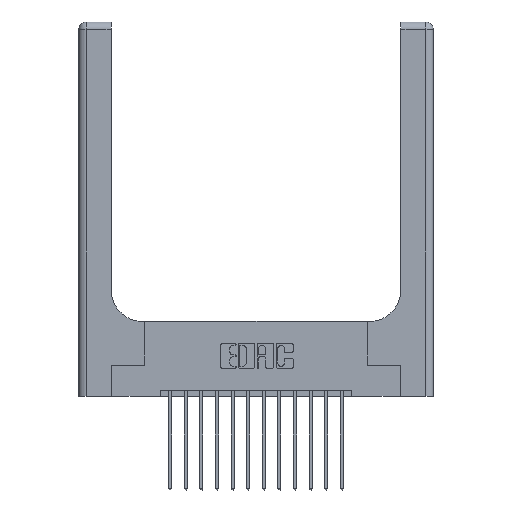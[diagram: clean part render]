
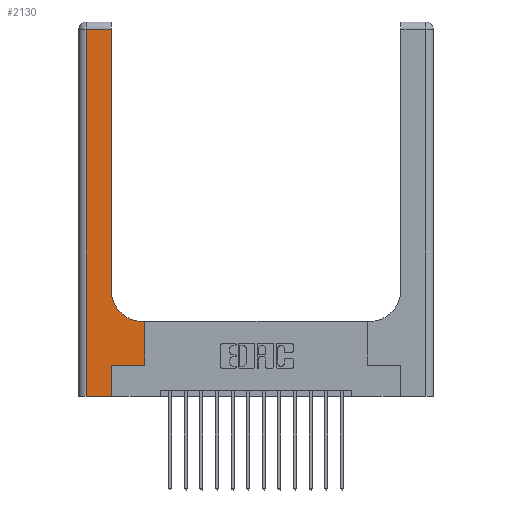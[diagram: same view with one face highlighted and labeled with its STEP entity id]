
A CAD part, top view. The second image highlights one B-rep face of the part: STEP entity #2130.
In plain terms, the highlighted planar face has unit normal (0, 0, 1).
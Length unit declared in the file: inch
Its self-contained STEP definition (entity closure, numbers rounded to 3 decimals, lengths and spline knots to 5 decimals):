
#129 = ORIENTED_EDGE ( 'NONE', *, *, #15152, .T. ) ;
#852 = DIRECTION ( 'NONE',  ( 0., -1., 0. ) ) ;
#1021 = VERTEX_POINT ( 'NONE', #17495 ) ;
#1095 = CARTESIAN_POINT ( 'NONE',  ( 0.26, 0.85, 0.37 ) ) ;
#1607 = DIRECTION ( 'NONE',  ( -1., 0., 0. ) ) ;
#1899 = EDGE_CURVE ( 'NONE', #12879, #5814, #5867, .T. ) ;
#1929 = LINE ( 'NONE', #7449, #6537 ) ;
#1983 = EDGE_CURVE ( 'NONE', #5428, #12879, #3203, .T. ) ;
#2092 = CARTESIAN_POINT ( 'NONE',  ( 0.06, 2.94, 0.37 ) ) ;
#2111 = DIRECTION ( 'NONE',  ( 0., 1., 0. ) ) ;
#2130 = ADVANCED_FACE ( 'NONE', ( #3716 ), #13783, .F. ) ;
#2487 = VECTOR ( 'NONE', #852, 39.37008 ) ;
#2728 = LINE ( 'NONE', #6643, #11378 ) ;
#3067 = DIRECTION ( 'NONE',  ( 1., 0., 0. ) ) ;
#3203 = LINE ( 'NONE', #8864, #11500 ) ;
#3237 = VERTEX_POINT ( 'NONE', #6046 ) ;
#3716 = FACE_OUTER_BOUND ( 'NONE', #5103, .T. ) ;
#3989 = VERTEX_POINT ( 'NONE', #14133 ) ;
#4398 = CARTESIAN_POINT ( 'NONE',  ( 0.265, 0., 0.37 ) ) ;
#4504 = ORIENTED_EDGE ( 'NONE', *, *, #11763, .T. ) ;
#4719 = DIRECTION ( 'NONE',  ( 0., 0., -1. ) ) ;
#4758 = AXIS2_PLACEMENT_3D ( 'NONE', #5479, #6899, #13527 ) ;
#4929 = EDGE_CURVE ( 'NONE', #3237, #6338, #2728, .T. ) ;
#5103 = EDGE_LOOP ( 'NONE', ( #14970, #12688, #16982, #13398, #15724, #7224, #9480, #4504, #129 ) ) ;
#5184 = CARTESIAN_POINT ( 'NONE',  ( 0.528, 0.6, 0.37 ) ) ;
#5428 = VERTEX_POINT ( 'NONE', #12118 ) ;
#5479 = CARTESIAN_POINT ( 'NONE',  ( 0., 3., 0.37 ) ) ;
#5552 = CARTESIAN_POINT ( 'NONE',  ( 0.265, 0.25, 0.37 ) ) ;
#5690 = CARTESIAN_POINT ( 'NONE',  ( 0.06, 3., 0.37 ) ) ;
#5814 = VERTEX_POINT ( 'NONE', #14232 ) ;
#5864 = CIRCLE ( 'NONE', #8407, 0.25 ) ;
#5867 = LINE ( 'NONE', #5690, #2487 ) ;
#6046 = CARTESIAN_POINT ( 'NONE',  ( 0.528, 0.25, 0.37 ) ) ;
#6338 = VERTEX_POINT ( 'NONE', #5184 ) ;
#6537 = VECTOR ( 'NONE', #2111, 39.37008 ) ;
#6643 = CARTESIAN_POINT ( 'NONE',  ( 0.528, 0.25, 0.37 ) ) ;
#6899 = DIRECTION ( 'NONE',  ( 0., 0., -1. ) ) ;
#7224 = ORIENTED_EDGE ( 'NONE', *, *, #11307, .T. ) ;
#7338 = VERTEX_POINT ( 'NONE', #11290 ) ;
#7449 = CARTESIAN_POINT ( 'NONE',  ( 0.26, 3., 0.37 ) ) ;
#7505 = EDGE_CURVE ( 'NONE', #5814, #7338, #8202, .T. ) ;
#8202 = LINE ( 'NONE', #16314, #13281 ) ;
#8407 = AXIS2_PLACEMENT_3D ( 'NONE', #16835, #4719, #15621 ) ;
#8470 = VECTOR ( 'NONE', #15561, 39.37008 ) ;
#8745 = LINE ( 'NONE', #4398, #8470 ) ;
#8864 = CARTESIAN_POINT ( 'NONE',  ( 0., 2.94, 0.37 ) ) ;
#9272 = VECTOR ( 'NONE', #3067, 39.37008 ) ;
#9480 = ORIENTED_EDGE ( 'NONE', *, *, #4929, .T. ) ;
#9571 = VECTOR ( 'NONE', #1607, 39.37008 ) ;
#9694 = LINE ( 'NONE', #13754, #9571 ) ;
#10663 = DIRECTION ( 'NONE',  ( 1., 0., 0. ) ) ;
#11290 = CARTESIAN_POINT ( 'NONE',  ( 0.265, 0., 0.37 ) ) ;
#11307 = EDGE_CURVE ( 'NONE', #1021, #3237, #16347, .T. ) ;
#11378 = VECTOR ( 'NONE', #16023, 39.37008 ) ;
#11500 = VECTOR ( 'NONE', #12407, 39.37008 ) ;
#11763 = EDGE_CURVE ( 'NONE', #6338, #3989, #9694, .T. ) ;
#12118 = CARTESIAN_POINT ( 'NONE',  ( 0.26, 2.94, 0.37 ) ) ;
#12407 = DIRECTION ( 'NONE',  ( -1., 0., 0. ) ) ;
#12688 = ORIENTED_EDGE ( 'NONE', *, *, #1983, .T. ) ;
#12879 = VERTEX_POINT ( 'NONE', #2092 ) ;
#12969 = VERTEX_POINT ( 'NONE', #1095 ) ;
#13281 = VECTOR ( 'NONE', #10663, 39.37008 ) ;
#13398 = ORIENTED_EDGE ( 'NONE', *, *, #7505, .T. ) ;
#13527 = DIRECTION ( 'NONE',  ( -1., 0., 0. ) ) ;
#13754 = CARTESIAN_POINT ( 'NONE',  ( 0.26, 0.6, 0.37 ) ) ;
#13783 = PLANE ( 'NONE',  #4758 ) ;
#14133 = CARTESIAN_POINT ( 'NONE',  ( 0.51, 0.6, 0.37 ) ) ;
#14232 = CARTESIAN_POINT ( 'NONE',  ( 0.06, 0., 0.37 ) ) ;
#14970 = ORIENTED_EDGE ( 'NONE', *, *, #17352, .T. ) ;
#15152 = EDGE_CURVE ( 'NONE', #3989, #12969, #5864, .T. ) ;
#15561 = DIRECTION ( 'NONE',  ( 0., 1., 0. ) ) ;
#15621 = DIRECTION ( 'NONE',  ( 1., 0., 0. ) ) ;
#15724 = ORIENTED_EDGE ( 'NONE', *, *, #16432, .T. ) ;
#16023 = DIRECTION ( 'NONE',  ( 0., 1., 0. ) ) ;
#16314 = CARTESIAN_POINT ( 'NONE',  ( 0., 0., 0.37 ) ) ;
#16347 = LINE ( 'NONE', #5552, #9272 ) ;
#16432 = EDGE_CURVE ( 'NONE', #7338, #1021, #8745, .T. ) ;
#16835 = CARTESIAN_POINT ( 'NONE',  ( 0.51, 0.85, 0.37 ) ) ;
#16982 = ORIENTED_EDGE ( 'NONE', *, *, #1899, .T. ) ;
#17352 = EDGE_CURVE ( 'NONE', #12969, #5428, #1929, .T. ) ;
#17495 = CARTESIAN_POINT ( 'NONE',  ( 0.265, 0.25, 0.37 ) ) ;
